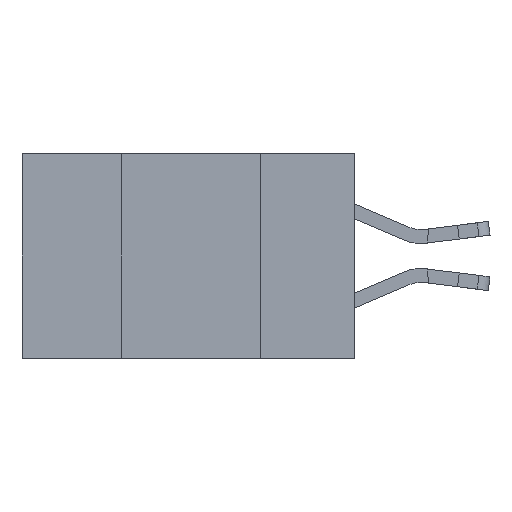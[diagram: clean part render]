
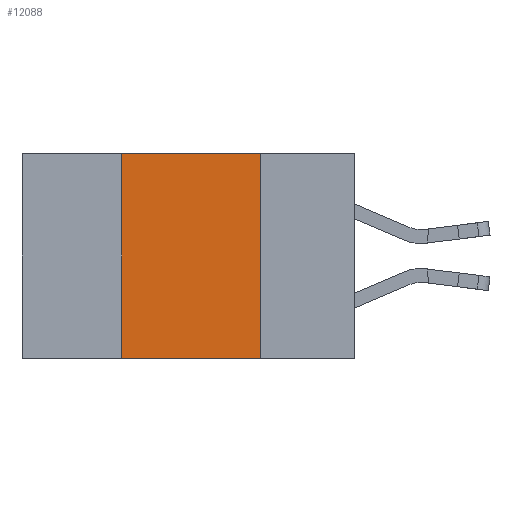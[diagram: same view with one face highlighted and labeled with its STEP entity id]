
A CAD part, left-side view. The second image highlights one B-rep face of the part: STEP entity #12088.
In plain terms, the highlighted planar face has unit normal (-1, 0, 0).
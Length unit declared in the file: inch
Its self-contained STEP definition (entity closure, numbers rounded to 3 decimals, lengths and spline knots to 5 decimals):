
#60 = EDGE_LOOP ( 'NONE', ( #6847, #4009, #8942, #8210 ) ) ;
#432 = LINE ( 'NONE', #3685, #11358 ) ;
#1277 = VECTOR ( 'NONE', #1665, 39.37008 ) ;
#1358 = CARTESIAN_POINT ( 'NONE',  ( 0., 0.17, -0.37 ) ) ;
#1604 = LINE ( 'NONE', #4763, #1277 ) ;
#1665 = DIRECTION ( 'NONE',  ( 0., 0., 1. ) ) ;
#1953 = EDGE_CURVE ( 'NONE', #1957, #8944, #432, .T. ) ;
#1957 = VERTEX_POINT ( 'NONE', #8993 ) ;
#3038 = DIRECTION ( 'NONE',  ( 0., -1., 0. ) ) ;
#3057 = VERTEX_POINT ( 'NONE', #7072 ) ;
#3685 = CARTESIAN_POINT ( 'NONE',  ( 0., 0.17, 0. ) ) ;
#4009 = ORIENTED_EDGE ( 'NONE', *, *, #4452, .F. ) ;
#4217 = FACE_OUTER_BOUND ( 'NONE', #60, .T. ) ;
#4452 = EDGE_CURVE ( 'NONE', #3057, #1957, #9807, .T. ) ;
#4763 = CARTESIAN_POINT ( 'NONE',  ( 0., 0.42, 0. ) ) ;
#4993 = PLANE ( 'NONE',  #13017 ) ;
#6031 = DIRECTION ( 'NONE',  ( 0., 0., -1. ) ) ;
#6501 = LINE ( 'NONE', #8367, #9059 ) ;
#6847 = ORIENTED_EDGE ( 'NONE', *, *, #1953, .F. ) ;
#7032 = CARTESIAN_POINT ( 'NONE',  ( 0., 0.6, 0. ) ) ;
#7072 = CARTESIAN_POINT ( 'NONE',  ( 0., 0.42, 0. ) ) ;
#7973 = VERTEX_POINT ( 'NONE', #12344 ) ;
#8210 = ORIENTED_EDGE ( 'NONE', *, *, #10894, .T. ) ;
#8367 = CARTESIAN_POINT ( 'NONE',  ( 0., 0.6, -0.37 ) ) ;
#8407 = DIRECTION ( 'NONE',  ( 0., 0., -1. ) ) ;
#8942 = ORIENTED_EDGE ( 'NONE', *, *, #11326, .F. ) ;
#8944 = VERTEX_POINT ( 'NONE', #1358 ) ;
#8993 = CARTESIAN_POINT ( 'NONE',  ( 0., 0.17, 0. ) ) ;
#9059 = VECTOR ( 'NONE', #3038, 39.37008 ) ;
#9807 = LINE ( 'NONE', #10330, #12899 ) ;
#10190 = DIRECTION ( 'NONE',  ( 0., -1., 0. ) ) ;
#10330 = CARTESIAN_POINT ( 'NONE',  ( 0., 0.6, 0. ) ) ;
#10894 = EDGE_CURVE ( 'NONE', #7973, #8944, #6501, .T. ) ;
#11326 = EDGE_CURVE ( 'NONE', #7973, #3057, #1604, .T. ) ;
#11358 = VECTOR ( 'NONE', #8407, 39.37008 ) ;
#12088 = ADVANCED_FACE ( 'NONE', ( #4217 ), #4993, .F. ) ;
#12344 = CARTESIAN_POINT ( 'NONE',  ( 0., 0.42, -0.37 ) ) ;
#12430 = DIRECTION ( 'NONE',  ( 1., 0., 0. ) ) ;
#12899 = VECTOR ( 'NONE', #10190, 39.37008 ) ;
#13017 = AXIS2_PLACEMENT_3D ( 'NONE', #7032, #12430, #6031 ) ;
